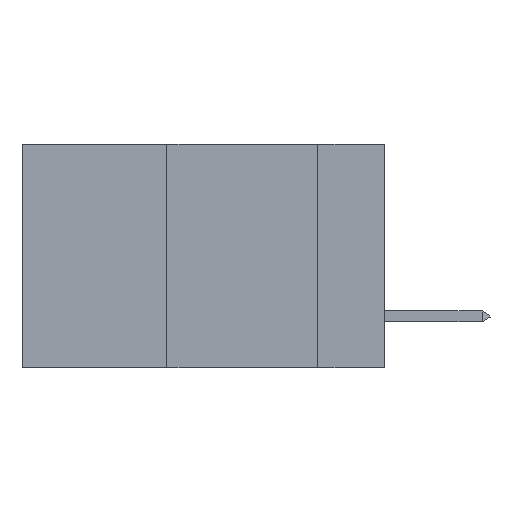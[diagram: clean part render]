
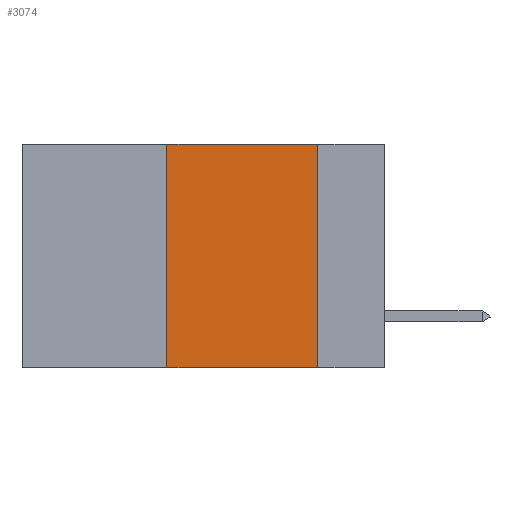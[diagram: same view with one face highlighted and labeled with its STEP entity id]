
A CAD part, left-side view. The second image highlights one B-rep face of the part: STEP entity #3074.
In plain terms, the highlighted planar face has unit normal (-1, 0, 0).
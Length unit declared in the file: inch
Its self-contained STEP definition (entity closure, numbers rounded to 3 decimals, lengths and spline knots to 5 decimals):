
#189 = EDGE_CURVE ( 'NONE', #9019, #12408, #15076, .T. ) ;
#316 = LINE ( 'NONE', #12906, #1259 ) ;
#687 = LINE ( 'NONE', #11255, #19121 ) ;
#835 = CARTESIAN_POINT ( 'NONE',  ( 0., 0.6, -0.37 ) ) ;
#1259 = VECTOR ( 'NONE', #10960, 39.37008 ) ;
#2896 = PLANE ( 'NONE',  #14399 ) ;
#3074 = ADVANCED_FACE ( 'NONE', ( #6178 ), #2896, .F. ) ;
#3980 = EDGE_CURVE ( 'NONE', #16676, #9019, #687, .T. ) ;
#4213 = ORIENTED_EDGE ( 'NONE', *, *, #189, .F. ) ;
#4510 = EDGE_LOOP ( 'NONE', ( #7841, #4213, #6833, #19238 ) ) ;
#4808 = DIRECTION ( 'NONE',  ( 0., 0., -1. ) ) ;
#4880 = VERTEX_POINT ( 'NONE', #24782 ) ;
#4886 = DIRECTION ( 'NONE',  ( 0., -1., 0. ) ) ;
#5118 = LINE ( 'NONE', #835, #21145 ) ;
#5287 = CARTESIAN_POINT ( 'NONE',  ( 0., 0.36, -0.37 ) ) ;
#6178 = FACE_OUTER_BOUND ( 'NONE', #4510, .T. ) ;
#6833 = ORIENTED_EDGE ( 'NONE', *, *, #3980, .F. ) ;
#7841 = ORIENTED_EDGE ( 'NONE', *, *, #16760, .F. ) ;
#8041 = DIRECTION ( 'NONE',  ( 0., 0., 1. ) ) ;
#8770 = DIRECTION ( 'NONE',  ( 0., -1., 0. ) ) ;
#9019 = VERTEX_POINT ( 'NONE', #16776 ) ;
#10960 = DIRECTION ( 'NONE',  ( 0., 0., -1. ) ) ;
#11255 = CARTESIAN_POINT ( 'NONE',  ( 0., 0.36, 0. ) ) ;
#11288 = EDGE_CURVE ( 'NONE', #16676, #4880, #5118, .T. ) ;
#12408 = VERTEX_POINT ( 'NONE', #24467 ) ;
#12906 = CARTESIAN_POINT ( 'NONE',  ( 0., 0.11, 0. ) ) ;
#14399 = AXIS2_PLACEMENT_3D ( 'NONE', #18233, #22398, #4808 ) ;
#15076 = LINE ( 'NONE', #23986, #24157 ) ;
#16676 = VERTEX_POINT ( 'NONE', #5287 ) ;
#16760 = EDGE_CURVE ( 'NONE', #12408, #4880, #316, .T. ) ;
#16776 = CARTESIAN_POINT ( 'NONE',  ( 0., 0.36, 0. ) ) ;
#18233 = CARTESIAN_POINT ( 'NONE',  ( 0., 0.6, 0. ) ) ;
#19121 = VECTOR ( 'NONE', #8041, 39.37008 ) ;
#19238 = ORIENTED_EDGE ( 'NONE', *, *, #11288, .T. ) ;
#21145 = VECTOR ( 'NONE', #4886, 39.37008 ) ;
#22398 = DIRECTION ( 'NONE',  ( 1., 0., 0. ) ) ;
#23986 = CARTESIAN_POINT ( 'NONE',  ( 0., 0.6, 0. ) ) ;
#24157 = VECTOR ( 'NONE', #8770, 39.37008 ) ;
#24467 = CARTESIAN_POINT ( 'NONE',  ( 0., 0.11, 0. ) ) ;
#24782 = CARTESIAN_POINT ( 'NONE',  ( 0., 0.11, -0.37 ) ) ;
